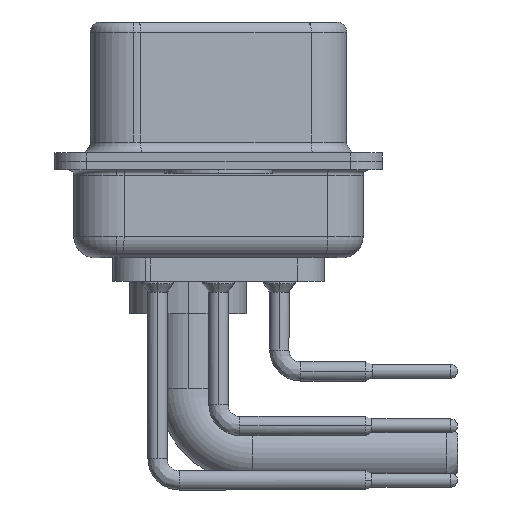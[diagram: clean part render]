
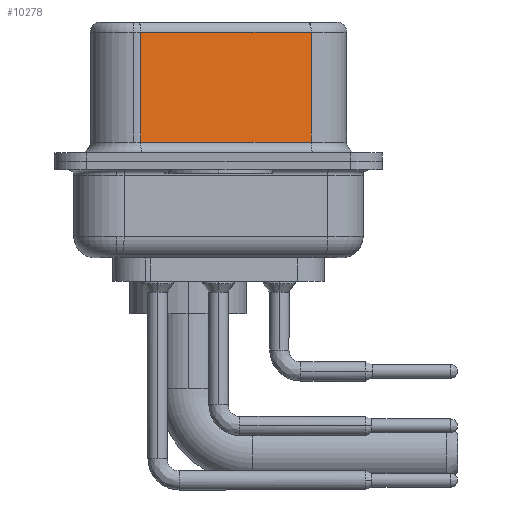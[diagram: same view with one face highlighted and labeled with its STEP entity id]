
A CAD part, left-side view. The second image highlights one B-rep face of the part: STEP entity #10278.
In plain terms, the highlighted planar face has unit normal (-0.985, -0.174, 0).
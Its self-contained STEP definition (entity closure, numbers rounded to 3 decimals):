
#1490 = AXIS2_PLACEMENT_3D ( 'NONE', #24780, #19375, #24956 ) ;
#2800 = CARTESIAN_POINT ( 'NONE',  ( 5.132, -4.322, 0.9 ) ) ;
#4494 = DIRECTION ( 'NONE',  ( 0., 0., -1. ) ) ;
#4931 = CARTESIAN_POINT ( 'NONE',  ( 3.73, 3.628, 6.02 ) ) ;
#5869 = LINE ( 'NONE', #2800, #20270 ) ;
#7062 = DIRECTION ( 'NONE',  ( 0., 0., -1. ) ) ;
#7547 = LINE ( 'NONE', #9900, #21567 ) ;
#8422 = DIRECTION ( 'NONE',  ( -0.174, 0.985, 0. ) ) ;
#9768 = LINE ( 'NONE', #26823, #24826 ) ;
#9900 = CARTESIAN_POINT ( 'NONE',  ( 5.132, -4.322, 6.52 ) ) ;
#10217 = ORIENTED_EDGE ( 'NONE', *, *, #17636, .T. ) ;
#10278 = ADVANCED_FACE ( 'NONE', ( #30011 ), #13997, .F. ) ;
#11272 = VERTEX_POINT ( 'NONE', #34011 ) ;
#11307 = CARTESIAN_POINT ( 'NONE',  ( 5.132, -4.322, 6.02 ) ) ;
#12528 = ORIENTED_EDGE ( 'NONE', *, *, #22132, .F. ) ;
#13624 = EDGE_LOOP ( 'NONE', ( #12528, #22239, #10217, #31469 ) ) ;
#13997 = PLANE ( 'NONE',  #1490 ) ;
#14791 = VERTEX_POINT ( 'NONE', #4931 ) ;
#15168 = VECTOR ( 'NONE', #8422, 1000. ) ;
#16306 = DIRECTION ( 'NONE',  ( 0.174, -0.985, 0. ) ) ;
#17636 = EDGE_CURVE ( 'NONE', #14791, #18067, #9768, .T. ) ;
#18067 = VERTEX_POINT ( 'NONE', #23916 ) ;
#19375 = DIRECTION ( 'NONE',  ( 0.985, 0.174, 0. ) ) ;
#20270 = VECTOR ( 'NONE', #16306, 1000. ) ;
#21567 = VECTOR ( 'NONE', #4494, 1000. ) ;
#22132 = EDGE_CURVE ( 'NONE', #34280, #11272, #7547, .T. ) ;
#22239 = ORIENTED_EDGE ( 'NONE', *, *, #33069, .T. ) ;
#23779 = CARTESIAN_POINT ( 'NONE',  ( 5.132, -4.322, 6.02 ) ) ;
#23916 = CARTESIAN_POINT ( 'NONE',  ( 3.73, 3.628, 0.9 ) ) ;
#24780 = CARTESIAN_POINT ( 'NONE',  ( 5.132, -4.322, 6.52 ) ) ;
#24826 = VECTOR ( 'NONE', #7062, 1000. ) ;
#24956 = DIRECTION ( 'NONE',  ( -0.174, 0.985, 0. ) ) ;
#24976 = LINE ( 'NONE', #11307, #15168 ) ;
#26823 = CARTESIAN_POINT ( 'NONE',  ( 3.73, 3.628, 6.52 ) ) ;
#30011 = FACE_OUTER_BOUND ( 'NONE', #13624, .T. ) ;
#31469 = ORIENTED_EDGE ( 'NONE', *, *, #32219, .T. ) ;
#32219 = EDGE_CURVE ( 'NONE', #18067, #11272, #5869, .T. ) ;
#33069 = EDGE_CURVE ( 'NONE', #34280, #14791, #24976, .T. ) ;
#34011 = CARTESIAN_POINT ( 'NONE',  ( 5.132, -4.322, 0.9 ) ) ;
#34280 = VERTEX_POINT ( 'NONE', #23779 ) ;
